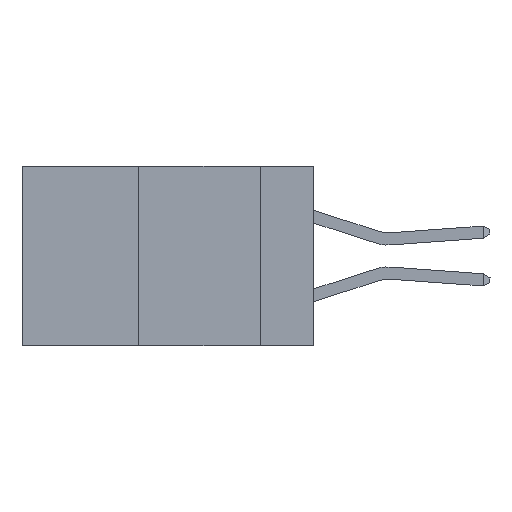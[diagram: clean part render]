
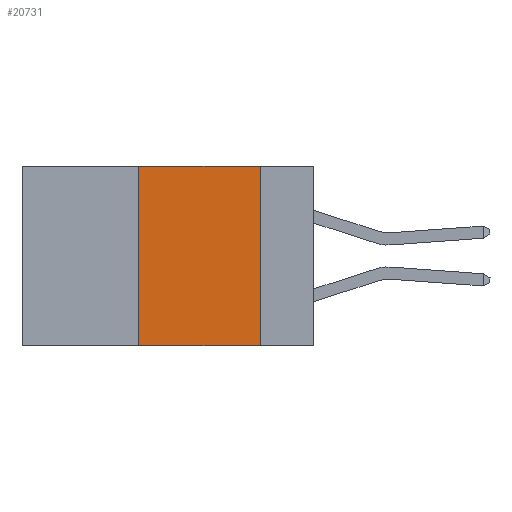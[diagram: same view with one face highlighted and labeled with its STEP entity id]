
A CAD part, left-side view. The second image highlights one B-rep face of the part: STEP entity #20731.
In plain terms, the highlighted planar face has unit normal (-1, 0, 0).
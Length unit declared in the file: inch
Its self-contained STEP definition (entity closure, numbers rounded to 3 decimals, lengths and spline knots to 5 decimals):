
#869 = LINE ( 'NONE', #15294, #11745 ) ;
#1562 = VERTEX_POINT ( 'NONE', #9861 ) ;
#2274 = ORIENTED_EDGE ( 'NONE', *, *, #22033, .F. ) ;
#2472 = FACE_OUTER_BOUND ( 'NONE', #4119, .T. ) ;
#3281 = EDGE_CURVE ( 'NONE', #24045, #1562, #23836, .T. ) ;
#4119 = EDGE_LOOP ( 'NONE', ( #19498, #18783, #2274, #24292 ) ) ;
#5743 = VECTOR ( 'NONE', #18158, 39.37008 ) ;
#5928 = DIRECTION ( 'NONE',  ( 0., 0., -1. ) ) ;
#6261 = DIRECTION ( 'NONE',  ( 1., 0., 0. ) ) ;
#6527 = PLANE ( 'NONE',  #11542 ) ;
#8091 = LINE ( 'NONE', #24029, #5743 ) ;
#8646 = LINE ( 'NONE', #10222, #22776 ) ;
#9861 = CARTESIAN_POINT ( 'NONE',  ( 0., 0.11, -0.37 ) ) ;
#10222 = CARTESIAN_POINT ( 'NONE',  ( 0., 0.36, 0. ) ) ;
#10991 = CARTESIAN_POINT ( 'NONE',  ( 0., 0.11, 0. ) ) ;
#11021 = VERTEX_POINT ( 'NONE', #19079 ) ;
#11542 = AXIS2_PLACEMENT_3D ( 'NONE', #22338, #6261, #20268 ) ;
#11745 = VECTOR ( 'NONE', #16858, 39.37008 ) ;
#13050 = CARTESIAN_POINT ( 'NONE',  ( 0., 0.36, 0. ) ) ;
#14101 = EDGE_CURVE ( 'NONE', #11021, #1562, #869, .T. ) ;
#15294 = CARTESIAN_POINT ( 'NONE',  ( 0., 0.6, -0.37 ) ) ;
#16084 = VERTEX_POINT ( 'NONE', #13050 ) ;
#16858 = DIRECTION ( 'NONE',  ( 0., -1., 0. ) ) ;
#18097 = CARTESIAN_POINT ( 'NONE',  ( 0., 0.11, 0. ) ) ;
#18158 = DIRECTION ( 'NONE',  ( 0., -1., 0. ) ) ;
#18783 = ORIENTED_EDGE ( 'NONE', *, *, #24342, .F. ) ;
#19079 = CARTESIAN_POINT ( 'NONE',  ( 0., 0.36, -0.37 ) ) ;
#19498 = ORIENTED_EDGE ( 'NONE', *, *, #3281, .F. ) ;
#20016 = DIRECTION ( 'NONE',  ( 0., 0., 1. ) ) ;
#20268 = DIRECTION ( 'NONE',  ( 0., 0., -1. ) ) ;
#20731 = ADVANCED_FACE ( 'NONE', ( #2472 ), #6527, .F. ) ;
#22033 = EDGE_CURVE ( 'NONE', #11021, #16084, #8646, .T. ) ;
#22338 = CARTESIAN_POINT ( 'NONE',  ( 0., 0.6, 0. ) ) ;
#22776 = VECTOR ( 'NONE', #20016, 39.37008 ) ;
#23836 = LINE ( 'NONE', #18097, #24398 ) ;
#24029 = CARTESIAN_POINT ( 'NONE',  ( 0., 0.6, 0. ) ) ;
#24045 = VERTEX_POINT ( 'NONE', #10991 ) ;
#24292 = ORIENTED_EDGE ( 'NONE', *, *, #14101, .T. ) ;
#24342 = EDGE_CURVE ( 'NONE', #16084, #24045, #8091, .T. ) ;
#24398 = VECTOR ( 'NONE', #5928, 39.37008 ) ;
